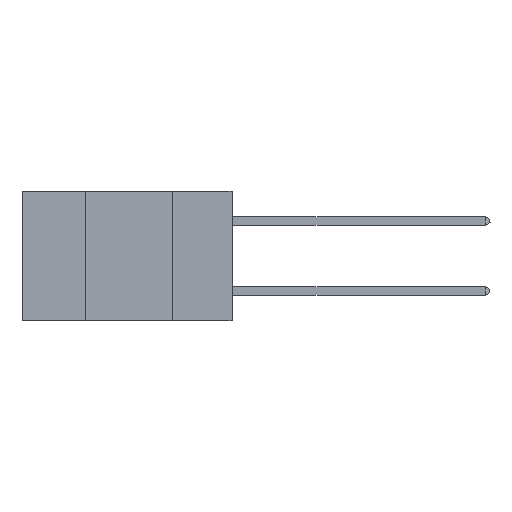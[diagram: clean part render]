
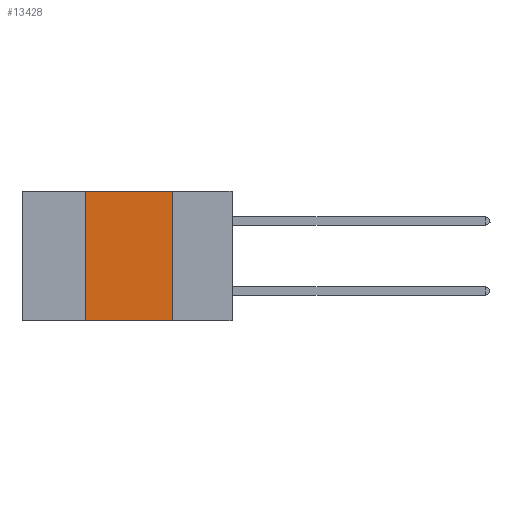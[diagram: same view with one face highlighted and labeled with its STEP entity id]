
A CAD part, left-side view. The second image highlights one B-rep face of the part: STEP entity #13428.
In plain terms, the highlighted planar face has unit normal (-1, 0, 0).
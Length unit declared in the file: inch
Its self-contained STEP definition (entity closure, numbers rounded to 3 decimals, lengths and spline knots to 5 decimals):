
#717 = ORIENTED_EDGE ( 'NONE', *, *, #13452, .F. ) ;
#2057 = EDGE_CURVE ( 'NONE', #8120, #20732, #13362, .T. ) ;
#3054 = VECTOR ( 'NONE', #22880, 39.37008 ) ;
#3978 = CARTESIAN_POINT ( 'NONE',  ( 0., 0.6, 0. ) ) ;
#4257 = VERTEX_POINT ( 'NONE', #24236 ) ;
#5380 = VERTEX_POINT ( 'NONE', #7042 ) ;
#5565 = ORIENTED_EDGE ( 'NONE', *, *, #24192, .F. ) ;
#6475 = LINE ( 'NONE', #23420, #12584 ) ;
#6822 = CARTESIAN_POINT ( 'NONE',  ( 0., 0.17, 0. ) ) ;
#7042 = CARTESIAN_POINT ( 'NONE',  ( 0., 0.17, -0.37 ) ) ;
#8120 = VERTEX_POINT ( 'NONE', #14415 ) ;
#8135 = CARTESIAN_POINT ( 'NONE',  ( 0., 0.17, 0. ) ) ;
#10348 = CARTESIAN_POINT ( 'NONE',  ( 0., 0.42, 0. ) ) ;
#12156 = DIRECTION ( 'NONE',  ( 0., -1., 0. ) ) ;
#12363 = EDGE_LOOP ( 'NONE', ( #5565, #18108, #717, #18959 ) ) ;
#12455 = FACE_OUTER_BOUND ( 'NONE', #12363, .T. ) ;
#12584 = VECTOR ( 'NONE', #12156, 39.37008 ) ;
#13362 = LINE ( 'NONE', #3978, #3054 ) ;
#13428 = ADVANCED_FACE ( 'NONE', ( #12455 ), #13930, .F. ) ;
#13452 = EDGE_CURVE ( 'NONE', #4257, #8120, #21961, .T. ) ;
#13930 = PLANE ( 'NONE',  #16598 ) ;
#14231 = VECTOR ( 'NONE', #23577, 39.37008 ) ;
#14304 = DIRECTION ( 'NONE',  ( 1., 0., 0. ) ) ;
#14415 = CARTESIAN_POINT ( 'NONE',  ( 0., 0.42, 0. ) ) ;
#16598 = AXIS2_PLACEMENT_3D ( 'NONE', #18000, #14304, #19981 ) ;
#18000 = CARTESIAN_POINT ( 'NONE',  ( 0., 0.6, 0. ) ) ;
#18108 = ORIENTED_EDGE ( 'NONE', *, *, #2057, .F. ) ;
#18959 = ORIENTED_EDGE ( 'NONE', *, *, #23761, .T. ) ;
#19981 = DIRECTION ( 'NONE',  ( 0., 0., -1. ) ) ;
#20732 = VERTEX_POINT ( 'NONE', #8135 ) ;
#21896 = DIRECTION ( 'NONE',  ( 0., 0., -1. ) ) ;
#21961 = LINE ( 'NONE', #10348, #14231 ) ;
#22861 = VECTOR ( 'NONE', #21896, 39.37008 ) ;
#22880 = DIRECTION ( 'NONE',  ( 0., -1., 0. ) ) ;
#23420 = CARTESIAN_POINT ( 'NONE',  ( 0., 0.6, -0.37 ) ) ;
#23577 = DIRECTION ( 'NONE',  ( 0., 0., 1. ) ) ;
#23761 = EDGE_CURVE ( 'NONE', #4257, #5380, #6475, .T. ) ;
#23770 = LINE ( 'NONE', #6822, #22861 ) ;
#24192 = EDGE_CURVE ( 'NONE', #20732, #5380, #23770, .T. ) ;
#24236 = CARTESIAN_POINT ( 'NONE',  ( 0., 0.42, -0.37 ) ) ;
